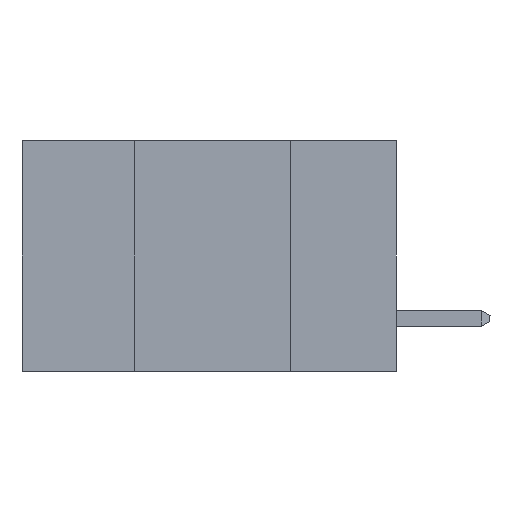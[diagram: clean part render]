
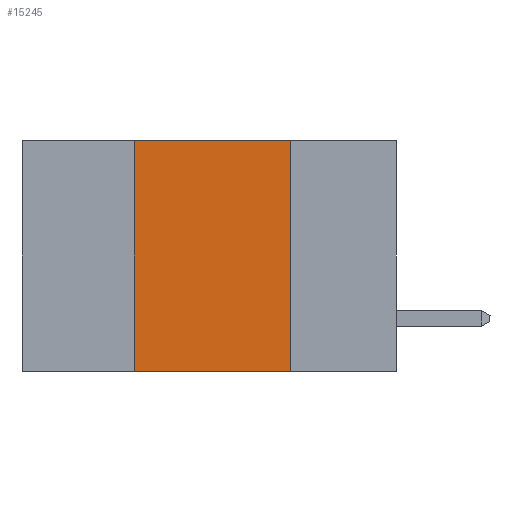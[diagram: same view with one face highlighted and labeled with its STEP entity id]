
A CAD part, left-side view. The second image highlights one B-rep face of the part: STEP entity #15245.
In plain terms, the highlighted planar face has unit normal (-1, 0, 0).
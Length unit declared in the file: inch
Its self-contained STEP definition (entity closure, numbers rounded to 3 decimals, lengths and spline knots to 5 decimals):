
#620 = AXIS2_PLACEMENT_3D ( 'NONE', #2691, #20545, #10677 ) ;
#787 = ORIENTED_EDGE ( 'NONE', *, *, #2678, .F. ) ;
#1295 = EDGE_CURVE ( 'NONE', #2265, #2368, #20095, .T. ) ;
#1980 = VERTEX_POINT ( 'NONE', #6889 ) ;
#2007 = CARTESIAN_POINT ( 'NONE',  ( 0., 0.42, 0. ) ) ;
#2265 = VERTEX_POINT ( 'NONE', #11193 ) ;
#2268 = VECTOR ( 'NONE', #9930, 39.37008 ) ;
#2302 = VECTOR ( 'NONE', #6672, 39.37008 ) ;
#2368 = VERTEX_POINT ( 'NONE', #11754 ) ;
#2678 = EDGE_CURVE ( 'NONE', #2265, #10006, #14759, .T. ) ;
#2691 = CARTESIAN_POINT ( 'NONE',  ( 0., 0.6, 0. ) ) ;
#4477 = FACE_OUTER_BOUND ( 'NONE', #15430, .T. ) ;
#6672 = DIRECTION ( 'NONE',  ( 0., 0., 1. ) ) ;
#6766 = ORIENTED_EDGE ( 'NONE', *, *, #1295, .T. ) ;
#6889 = CARTESIAN_POINT ( 'NONE',  ( 0., 0.17, 0. ) ) ;
#7402 = CARTESIAN_POINT ( 'NONE',  ( 0., 0.6, -0.37 ) ) ;
#8054 = CARTESIAN_POINT ( 'NONE',  ( 0., 0.6, 0. ) ) ;
#8840 = DIRECTION ( 'NONE',  ( 0., 0., -1. ) ) ;
#9930 = DIRECTION ( 'NONE',  ( 0., -1., 0. ) ) ;
#9999 = VECTOR ( 'NONE', #8840, 39.37008 ) ;
#10006 = VERTEX_POINT ( 'NONE', #2007 ) ;
#10677 = DIRECTION ( 'NONE',  ( 0., 0., -1. ) ) ;
#10887 = PLANE ( 'NONE',  #620 ) ;
#11193 = CARTESIAN_POINT ( 'NONE',  ( 0., 0.42, -0.37 ) ) ;
#11308 = LINE ( 'NONE', #8054, #2268 ) ;
#11754 = CARTESIAN_POINT ( 'NONE',  ( 0., 0.17, -0.37 ) ) ;
#12642 = EDGE_CURVE ( 'NONE', #1980, #2368, #18475, .T. ) ;
#13304 = EDGE_CURVE ( 'NONE', #10006, #1980, #11308, .T. ) ;
#14653 = CARTESIAN_POINT ( 'NONE',  ( 0., 0.42, -0.37 ) ) ;
#14759 = LINE ( 'NONE', #14653, #2302 ) ;
#15245 = ADVANCED_FACE ( 'NONE', ( #4477 ), #10887, .F. ) ;
#15430 = EDGE_LOOP ( 'NONE', ( #20302, #16230, #787, #6766 ) ) ;
#16230 = ORIENTED_EDGE ( 'NONE', *, *, #13304, .F. ) ;
#17011 = VECTOR ( 'NONE', #18304, 39.37008 ) ;
#18304 = DIRECTION ( 'NONE',  ( 0., -1., 0. ) ) ;
#18475 = LINE ( 'NONE', #20051, #9999 ) ;
#20051 = CARTESIAN_POINT ( 'NONE',  ( 0., 0.17, -0.37 ) ) ;
#20095 = LINE ( 'NONE', #7402, #17011 ) ;
#20302 = ORIENTED_EDGE ( 'NONE', *, *, #12642, .F. ) ;
#20545 = DIRECTION ( 'NONE',  ( 1., 0., 0. ) ) ;
